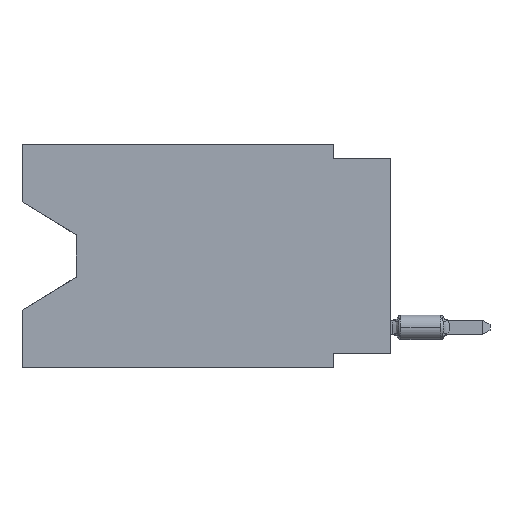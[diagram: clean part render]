
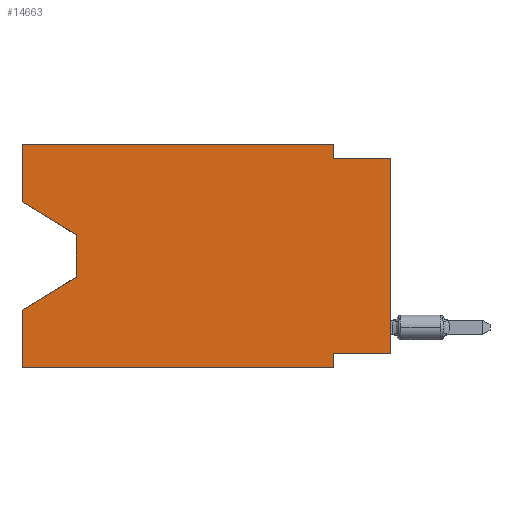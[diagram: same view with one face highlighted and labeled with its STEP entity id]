
A CAD part, left-side view. The second image highlights one B-rep face of the part: STEP entity #14663.
In plain terms, the highlighted planar face has unit normal (-1, 0, 0).
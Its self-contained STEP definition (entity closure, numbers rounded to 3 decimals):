
#32 = LINE ( 'NONE', #4816, #15195 ) ;
#90 = VECTOR ( 'NONE', #5661, 1000. ) ;
#214 = VERTEX_POINT ( 'NONE', #7446 ) ;
#220 = ORIENTED_EDGE ( 'NONE', *, *, #8831, .T. ) ;
#252 = EDGE_CURVE ( 'NONE', #10909, #15016, #3275, .T. ) ;
#372 = VECTOR ( 'NONE', #8088, 1000. ) ;
#625 = CARTESIAN_POINT ( 'NONE',  ( 0., 0., 0. ) ) ;
#705 = DIRECTION ( 'NONE',  ( 0., 0., -1. ) ) ;
#730 = EDGE_CURVE ( 'NONE', #8265, #12503, #1900, .T. ) ;
#756 = CARTESIAN_POINT ( 'NONE',  ( 0., 16.383, 0. ) ) ;
#758 = CARTESIAN_POINT ( 'NONE',  ( 0., 2.54, -0.635 ) ) ;
#815 = LINE ( 'NONE', #10494, #5319 ) ;
#899 = DIRECTION ( 'NONE',  ( 0., 0., -1. ) ) ;
#1045 = CARTESIAN_POINT ( 'NONE',  ( 0., 13.97, -5.893 ) ) ;
#1207 = LINE ( 'NONE', #8365, #7618 ) ;
#1900 = LINE ( 'NONE', #10170, #9418 ) ;
#2133 = ORIENTED_EDGE ( 'NONE', *, *, #8250, .F. ) ;
#2365 = EDGE_CURVE ( 'NONE', #214, #12503, #815, .T. ) ;
#2435 = LINE ( 'NONE', #6045, #4893 ) ;
#2983 = DIRECTION ( 'NONE',  ( 1., 0., 0. ) ) ;
#3062 = VECTOR ( 'NONE', #7670, 1000. ) ;
#3275 = LINE ( 'NONE', #11713, #372 ) ;
#3535 = ORIENTED_EDGE ( 'NONE', *, *, #730, .T. ) ;
#3557 = CARTESIAN_POINT ( 'NONE',  ( 0., 0., -9.271 ) ) ;
#4084 = VERTEX_POINT ( 'NONE', #7094 ) ;
#4125 = EDGE_LOOP ( 'NONE', ( #7781, #5459, #4936, #13872, #3535, #4448, #10283, #220, #5802, #2133, #8097, #14561 ) ) ;
#4196 = VECTOR ( 'NONE', #11915, 1000. ) ;
#4200 = LINE ( 'NONE', #5521, #3062 ) ;
#4364 = EDGE_CURVE ( 'NONE', #5203, #4084, #5435, .T. ) ;
#4448 = ORIENTED_EDGE ( 'NONE', *, *, #2365, .F. ) ;
#4565 = CARTESIAN_POINT ( 'NONE',  ( 0., 16.383, -9.906 ) ) ;
#4816 = CARTESIAN_POINT ( 'NONE',  ( 0., 16.383, -2.546 ) ) ;
#4893 = VECTOR ( 'NONE', #10700, 1000. ) ;
#4936 = ORIENTED_EDGE ( 'NONE', *, *, #11877, .T. ) ;
#5203 = VERTEX_POINT ( 'NONE', #758 ) ;
#5319 = VECTOR ( 'NONE', #899, 1000. ) ;
#5366 = DIRECTION ( 'NONE',  ( 0., -1., 0. ) ) ;
#5435 = LINE ( 'NONE', #10380, #90 ) ;
#5459 = ORIENTED_EDGE ( 'NONE', *, *, #6972, .T. ) ;
#5521 = CARTESIAN_POINT ( 'NONE',  ( 0., 13.97, -4.013 ) ) ;
#5661 = DIRECTION ( 'NONE',  ( 0., -1., 0. ) ) ;
#5736 = LINE ( 'NONE', #10542, #8460 ) ;
#5802 = ORIENTED_EDGE ( 'NONE', *, *, #4364, .F. ) ;
#6045 = CARTESIAN_POINT ( 'NONE',  ( 0., 0., -9.271 ) ) ;
#6703 = EDGE_CURVE ( 'NONE', #10909, #12726, #32, .T. ) ;
#6869 = DIRECTION ( 'NONE',  ( 0., -0.855, -0.519 ) ) ;
#6972 = EDGE_CURVE ( 'NONE', #12726, #8663, #4200, .T. ) ;
#7094 = CARTESIAN_POINT ( 'NONE',  ( 0., 0., -0.635 ) ) ;
#7187 = DIRECTION ( 'NONE',  ( 0., 0., -1. ) ) ;
#7233 = CARTESIAN_POINT ( 'NONE',  ( 0., 16.383, 0. ) ) ;
#7446 = CARTESIAN_POINT ( 'NONE',  ( 0., 2.54, -9.271 ) ) ;
#7618 = VECTOR ( 'NONE', #7187, 1000. ) ;
#7670 = DIRECTION ( 'NONE',  ( 0., 0., -1. ) ) ;
#7686 = LINE ( 'NONE', #7233, #10699 ) ;
#7781 = ORIENTED_EDGE ( 'NONE', *, *, #6703, .T. ) ;
#7787 = PLANE ( 'NONE',  #13459 ) ;
#7832 = VERTEX_POINT ( 'NONE', #14356 ) ;
#7866 = CARTESIAN_POINT ( 'NONE',  ( 0., 13.97, -4.013 ) ) ;
#8088 = DIRECTION ( 'NONE',  ( 0., 0., 1. ) ) ;
#8097 = ORIENTED_EDGE ( 'NONE', *, *, #12873, .F. ) ;
#8132 = LINE ( 'NONE', #1045, #4196 ) ;
#8250 = EDGE_CURVE ( 'NONE', #12499, #5203, #1207, .T. ) ;
#8265 = VERTEX_POINT ( 'NONE', #4565 ) ;
#8365 = CARTESIAN_POINT ( 'NONE',  ( 0., 2.54, 0. ) ) ;
#8460 = VECTOR ( 'NONE', #15338, 1000. ) ;
#8663 = VERTEX_POINT ( 'NONE', #14326 ) ;
#8831 = EDGE_CURVE ( 'NONE', #9386, #4084, #14872, .T. ) ;
#8882 = FACE_OUTER_BOUND ( 'NONE', #4125, .T. ) ;
#9386 = VERTEX_POINT ( 'NONE', #3557 ) ;
#9418 = VECTOR ( 'NONE', #5366, 1000. ) ;
#10036 = DIRECTION ( 'NONE',  ( 0., -1., 0. ) ) ;
#10170 = CARTESIAN_POINT ( 'NONE',  ( 0., 16.383, -9.906 ) ) ;
#10283 = ORIENTED_EDGE ( 'NONE', *, *, #14500, .F. ) ;
#10380 = CARTESIAN_POINT ( 'NONE',  ( 0., 0., -0.635 ) ) ;
#10494 = CARTESIAN_POINT ( 'NONE',  ( 0., 2.54, -9.906 ) ) ;
#10542 = CARTESIAN_POINT ( 'NONE',  ( 0., 16.383, 0. ) ) ;
#10648 = VECTOR ( 'NONE', #11323, 1000. ) ;
#10699 = VECTOR ( 'NONE', #10036, 1000. ) ;
#10700 = DIRECTION ( 'NONE',  ( 0., 1., 0. ) ) ;
#10909 = VERTEX_POINT ( 'NONE', #11042 ) ;
#11042 = CARTESIAN_POINT ( 'NONE',  ( 0., 16.383, -2.546 ) ) ;
#11323 = DIRECTION ( 'NONE',  ( 0., 0., 1. ) ) ;
#11713 = CARTESIAN_POINT ( 'NONE',  ( 0., 16.383, 0. ) ) ;
#11877 = EDGE_CURVE ( 'NONE', #8663, #7832, #8132, .T. ) ;
#11915 = DIRECTION ( 'NONE',  ( 0., 0.855, -0.519 ) ) ;
#12499 = VERTEX_POINT ( 'NONE', #13474 ) ;
#12503 = VERTEX_POINT ( 'NONE', #14643 ) ;
#12726 = VERTEX_POINT ( 'NONE', #7866 ) ;
#12873 = EDGE_CURVE ( 'NONE', #15016, #12499, #7686, .T. ) ;
#13444 = EDGE_CURVE ( 'NONE', #8265, #7832, #5736, .T. ) ;
#13459 = AXIS2_PLACEMENT_3D ( 'NONE', #13770, #2983, #705 ) ;
#13474 = CARTESIAN_POINT ( 'NONE',  ( 0., 2.54, 0. ) ) ;
#13770 = CARTESIAN_POINT ( 'NONE',  ( 0., 16.383, 0. ) ) ;
#13872 = ORIENTED_EDGE ( 'NONE', *, *, #13444, .F. ) ;
#14326 = CARTESIAN_POINT ( 'NONE',  ( 0., 13.97, -5.893 ) ) ;
#14356 = CARTESIAN_POINT ( 'NONE',  ( 0., 16.383, -7.36 ) ) ;
#14500 = EDGE_CURVE ( 'NONE', #9386, #214, #2435, .T. ) ;
#14561 = ORIENTED_EDGE ( 'NONE', *, *, #252, .F. ) ;
#14643 = CARTESIAN_POINT ( 'NONE',  ( 0., 2.54, -9.906 ) ) ;
#14663 = ADVANCED_FACE ( 'NONE', ( #8882 ), #7787, .F. ) ;
#14872 = LINE ( 'NONE', #625, #10648 ) ;
#15016 = VERTEX_POINT ( 'NONE', #756 ) ;
#15195 = VECTOR ( 'NONE', #6869, 1000. ) ;
#15338 = DIRECTION ( 'NONE',  ( 0., 0., 1. ) ) ;
